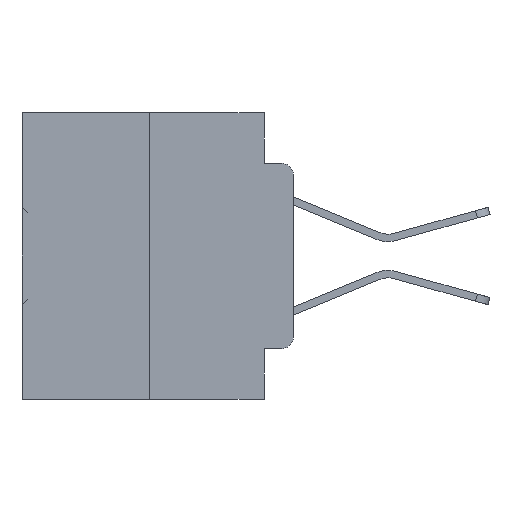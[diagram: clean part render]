
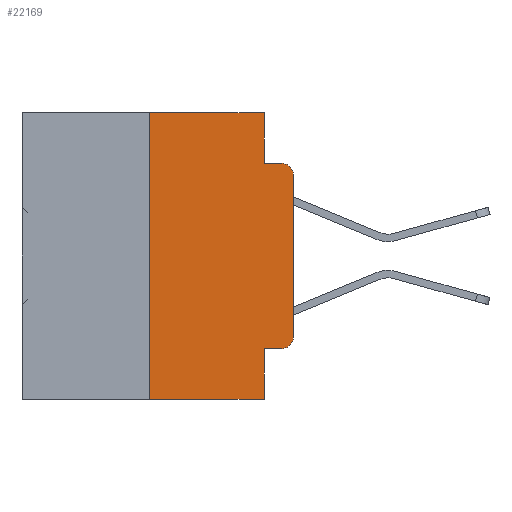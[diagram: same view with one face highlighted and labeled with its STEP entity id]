
A CAD part, left-side view. The second image highlights one B-rep face of the part: STEP entity #22169.
In plain terms, the highlighted planar face has unit normal (-1, 0, 0).
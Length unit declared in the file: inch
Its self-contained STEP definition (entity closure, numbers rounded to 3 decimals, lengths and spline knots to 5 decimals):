
#1375 = ORIENTED_EDGE ( 'NONE', *, *, #6358, .F. ) ;
#3548 = ORIENTED_EDGE ( 'NONE', *, *, #38605, .F. ) ;
#4445 = CARTESIAN_POINT ( 'NONE',  ( 0., 0.051, -0.4115 ) ) ;
#5014 = VERTEX_POINT ( 'NONE', #17272 ) ;
#5119 = DIRECTION ( 'NONE',  ( 1., 0., 0. ) ) ;
#5360 = ORIENTED_EDGE ( 'NONE', *, *, #10685, .T. ) ;
#5660 = ORIENTED_EDGE ( 'NONE', *, *, #34950, .F. ) ;
#5717 = CARTESIAN_POINT ( 'NONE',  ( 0., 0.051, -0.0885 ) ) ;
#5975 = LINE ( 'NONE', #19065, #20748 ) ;
#6315 = CARTESIAN_POINT ( 'NONE',  ( 0., 0.051, 0. ) ) ;
#6358 = EDGE_CURVE ( 'NONE', #13730, #25080, #13381, .T. ) ;
#6820 = VECTOR ( 'NONE', #32207, 39.37008 ) ;
#6884 = VECTOR ( 'NONE', #19037, 39.37008 ) ;
#7099 = VERTEX_POINT ( 'NONE', #7348 ) ;
#7348 = CARTESIAN_POINT ( 'NONE',  ( 0., 0.02, -0.4115 ) ) ;
#8813 = VERTEX_POINT ( 'NONE', #17115 ) ;
#9024 = DIRECTION ( 'NONE',  ( 0., -1., 0. ) ) ;
#9069 = DIRECTION ( 'NONE',  ( 0., 0., -1. ) ) ;
#9230 = CARTESIAN_POINT ( 'NONE',  ( 0., 0.25, 0. ) ) ;
#9669 = LINE ( 'NONE', #6315, #22487 ) ;
#10138 = EDGE_CURVE ( 'NONE', #25753, #36718, #5975, .T. ) ;
#10678 = CARTESIAN_POINT ( 'NONE',  ( 0., 0.051, 0. ) ) ;
#10685 = EDGE_CURVE ( 'NONE', #25753, #33552, #23544, .T. ) ;
#11472 = CARTESIAN_POINT ( 'NONE',  ( 0., 0.02, -0.1085 ) ) ;
#11852 = ORIENTED_EDGE ( 'NONE', *, *, #26208, .T. ) ;
#11936 = VERTEX_POINT ( 'NONE', #4445 ) ;
#12371 = CARTESIAN_POINT ( 'NONE',  ( 0., 0.051, 0. ) ) ;
#12773 = DIRECTION ( 'NONE',  ( 0., -1., 0. ) ) ;
#13381 = LINE ( 'NONE', #12371, #19105 ) ;
#13730 = VERTEX_POINT ( 'NONE', #10678 ) ;
#14380 = VECTOR ( 'NONE', #12773, 39.37008 ) ;
#15868 = CARTESIAN_POINT ( 'NONE',  ( 0., 0.051, -0.4115 ) ) ;
#17115 = CARTESIAN_POINT ( 'NONE',  ( 0., 0.02, -0.0885 ) ) ;
#17272 = CARTESIAN_POINT ( 'NONE',  ( 0., 0., -0.3915 ) ) ;
#17595 = CARTESIAN_POINT ( 'NONE',  ( 0., 0.473, 0. ) ) ;
#18369 = CARTESIAN_POINT ( 'NONE',  ( 0., 0.02, -0.3915 ) ) ;
#19022 = CARTESIAN_POINT ( 'NONE',  ( 0., 0.473, -0.5 ) ) ;
#19037 = DIRECTION ( 'NONE',  ( 0., -1., 0. ) ) ;
#19065 = CARTESIAN_POINT ( 'NONE',  ( 0., 0.25, 0. ) ) ;
#19105 = VECTOR ( 'NONE', #27168, 39.37008 ) ;
#19749 = LINE ( 'NONE', #15868, #6884 ) ;
#20535 = DIRECTION ( 'NONE',  ( 0., 0., -1. ) ) ;
#20745 = ORIENTED_EDGE ( 'NONE', *, *, #39263, .F. ) ;
#20748 = VECTOR ( 'NONE', #37689, 39.37008 ) ;
#21063 = DIRECTION ( 'NONE',  ( -1., 0., 0. ) ) ;
#22169 = ADVANCED_FACE ( 'NONE', ( #35950 ), #32752, .F. ) ;
#22487 = VECTOR ( 'NONE', #24684, 39.37008 ) ;
#22723 = EDGE_CURVE ( 'NONE', #11936, #7099, #19749, .T. ) ;
#23544 = LINE ( 'NONE', #19022, #37773 ) ;
#23916 = ORIENTED_EDGE ( 'NONE', *, *, #10138, .F. ) ;
#24684 = DIRECTION ( 'NONE',  ( 0., 0., -1. ) ) ;
#25080 = VERTEX_POINT ( 'NONE', #26735 ) ;
#25305 = CARTESIAN_POINT ( 'NONE',  ( 0., 0.051, -0.5 ) ) ;
#25441 = EDGE_LOOP ( 'NONE', ( #11852, #32242, #5660, #1375, #20745, #23916, #5360, #3548, #27083, #34024 ) ) ;
#25753 = VERTEX_POINT ( 'NONE', #30003 ) ;
#25883 = LINE ( 'NONE', #38482, #6820 ) ;
#26208 = EDGE_CURVE ( 'NONE', #5014, #32457, #25883, .T. ) ;
#26735 = CARTESIAN_POINT ( 'NONE',  ( 0., 0.051, -0.0885 ) ) ;
#26760 = LINE ( 'NONE', #33782, #14380 ) ;
#27083 = ORIENTED_EDGE ( 'NONE', *, *, #22723, .T. ) ;
#27112 = CIRCLE ( 'NONE', #38754, 0.02 ) ;
#27168 = DIRECTION ( 'NONE',  ( 0., 0., -1. ) ) ;
#28070 = AXIS2_PLACEMENT_3D ( 'NONE', #18369, #36969, #9069 ) ;
#28076 = CARTESIAN_POINT ( 'NONE',  ( 0., 0., -0.1085 ) ) ;
#28220 = DIRECTION ( 'NONE',  ( 0., -1., 0. ) ) ;
#29106 = VECTOR ( 'NONE', #9024, 39.37008 ) ;
#29603 = AXIS2_PLACEMENT_3D ( 'NONE', #17595, #5119, #35644 ) ;
#30003 = CARTESIAN_POINT ( 'NONE',  ( 0., 0.25, -0.5 ) ) ;
#32041 = EDGE_CURVE ( 'NONE', #32457, #8813, #27112, .T. ) ;
#32207 = DIRECTION ( 'NONE',  ( 0., 0., 1. ) ) ;
#32242 = ORIENTED_EDGE ( 'NONE', *, *, #32041, .T. ) ;
#32457 = VERTEX_POINT ( 'NONE', #28076 ) ;
#32752 = PLANE ( 'NONE',  #29603 ) ;
#32912 = CIRCLE ( 'NONE', #28070, 0.02 ) ;
#33552 = VERTEX_POINT ( 'NONE', #25305 ) ;
#33782 = CARTESIAN_POINT ( 'NONE',  ( 0., 0.473, 0. ) ) ;
#34024 = ORIENTED_EDGE ( 'NONE', *, *, #34319, .T. ) ;
#34319 = EDGE_CURVE ( 'NONE', #7099, #5014, #32912, .T. ) ;
#34950 = EDGE_CURVE ( 'NONE', #25080, #8813, #35747, .T. ) ;
#35644 = DIRECTION ( 'NONE',  ( 0., 0., -1. ) ) ;
#35747 = LINE ( 'NONE', #5717, #29106 ) ;
#35950 = FACE_OUTER_BOUND ( 'NONE', #25441, .T. ) ;
#36718 = VERTEX_POINT ( 'NONE', #9230 ) ;
#36969 = DIRECTION ( 'NONE',  ( -1., 0., 0. ) ) ;
#37689 = DIRECTION ( 'NONE',  ( 0., 0., 1. ) ) ;
#37773 = VECTOR ( 'NONE', #28220, 39.37008 ) ;
#38482 = CARTESIAN_POINT ( 'NONE',  ( 0., 0., 0. ) ) ;
#38605 = EDGE_CURVE ( 'NONE', #11936, #33552, #9669, .T. ) ;
#38754 = AXIS2_PLACEMENT_3D ( 'NONE', #11472, #21063, #20535 ) ;
#39263 = EDGE_CURVE ( 'NONE', #36718, #13730, #26760, .T. ) ;
